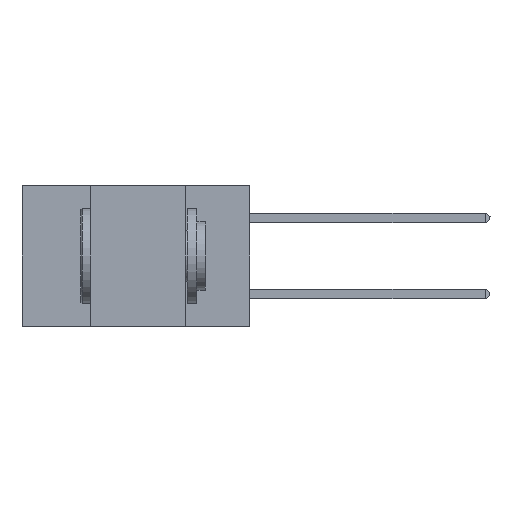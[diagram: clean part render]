
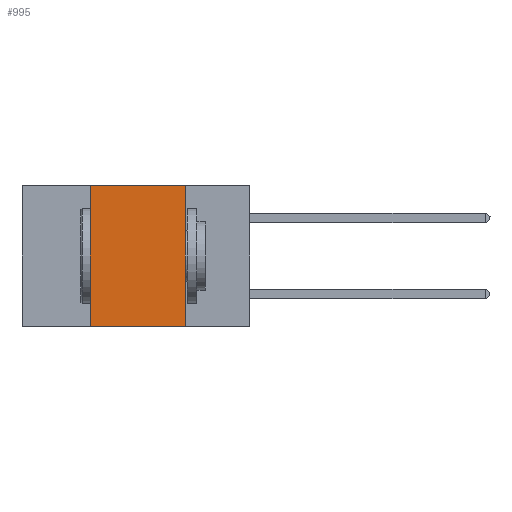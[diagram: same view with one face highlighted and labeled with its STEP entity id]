
A CAD part, left-side view. The second image highlights one B-rep face of the part: STEP entity #995.
In plain terms, the highlighted planar face has unit normal (-1, 0, 0).
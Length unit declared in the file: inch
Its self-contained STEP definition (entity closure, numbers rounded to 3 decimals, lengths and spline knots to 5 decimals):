
#995 = ADVANCED_FACE ( 'NONE', ( #11524 ), #20490, .F. ) ;
#2411 = CARTESIAN_POINT ( 'NONE',  ( 0., 0.17, 0. ) ) ;
#3609 = VERTEX_POINT ( 'NONE', #12390 ) ;
#3703 = DIRECTION ( 'NONE',  ( 0., -1., 0. ) ) ;
#4895 = CARTESIAN_POINT ( 'NONE',  ( 0., 0.17, 0. ) ) ;
#5444 = VECTOR ( 'NONE', #3703, 39.37008 ) ;
#5458 = EDGE_CURVE ( 'NONE', #3609, #16895, #18400, .T. ) ;
#5533 = DIRECTION ( 'NONE',  ( 0., 0., -1. ) ) ;
#6070 = ORIENTED_EDGE ( 'NONE', *, *, #5458, .F. ) ;
#6563 = AXIS2_PLACEMENT_3D ( 'NONE', #7487, #14064, #5533 ) ;
#7487 = CARTESIAN_POINT ( 'NONE',  ( 0., 0.6, 0. ) ) ;
#9781 = CARTESIAN_POINT ( 'NONE',  ( 0., 0.6, 0. ) ) ;
#11524 = FACE_OUTER_BOUND ( 'NONE', #19662, .T. ) ;
#12390 = CARTESIAN_POINT ( 'NONE',  ( 0., 0.42, 0. ) ) ;
#13765 = CARTESIAN_POINT ( 'NONE',  ( 0., 0.17, -0.37 ) ) ;
#14064 = DIRECTION ( 'NONE',  ( 1., 0., 0. ) ) ;
#14244 = CARTESIAN_POINT ( 'NONE',  ( 0., 0.42, 0. ) ) ;
#14337 = DIRECTION ( 'NONE',  ( 0., 0., 1. ) ) ;
#14833 = ORIENTED_EDGE ( 'NONE', *, *, #24848, .T. ) ;
#15168 = VECTOR ( 'NONE', #14337, 39.37008 ) ;
#16895 = VERTEX_POINT ( 'NONE', #2411 ) ;
#17498 = LINE ( 'NONE', #4895, #26363 ) ;
#18280 = LINE ( 'NONE', #27333, #5444 ) ;
#18400 = LINE ( 'NONE', #9781, #24902 ) ;
#18423 = ORIENTED_EDGE ( 'NONE', *, *, #19428, .F. ) ;
#18582 = VERTEX_POINT ( 'NONE', #25674 ) ;
#19428 = EDGE_CURVE ( 'NONE', #18582, #3609, #26772, .T. ) ;
#19662 = EDGE_LOOP ( 'NONE', ( #21610, #6070, #18423, #14833 ) ) ;
#20322 = EDGE_CURVE ( 'NONE', #16895, #27446, #17498, .T. ) ;
#20490 = PLANE ( 'NONE',  #6563 ) ;
#21610 = ORIENTED_EDGE ( 'NONE', *, *, #20322, .F. ) ;
#24520 = DIRECTION ( 'NONE',  ( 0., 0., -1. ) ) ;
#24848 = EDGE_CURVE ( 'NONE', #18582, #27446, #18280, .T. ) ;
#24902 = VECTOR ( 'NONE', #26985, 39.37008 ) ;
#25674 = CARTESIAN_POINT ( 'NONE',  ( 0., 0.42, -0.37 ) ) ;
#26363 = VECTOR ( 'NONE', #24520, 39.37008 ) ;
#26772 = LINE ( 'NONE', #14244, #15168 ) ;
#26985 = DIRECTION ( 'NONE',  ( 0., -1., 0. ) ) ;
#27333 = CARTESIAN_POINT ( 'NONE',  ( 0., 0.6, -0.37 ) ) ;
#27446 = VERTEX_POINT ( 'NONE', #13765 ) ;
